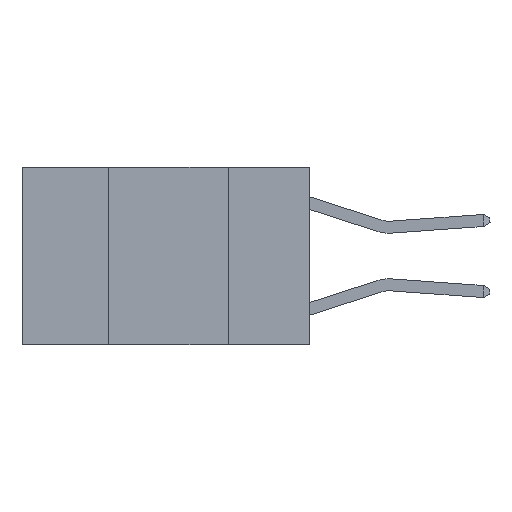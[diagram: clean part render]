
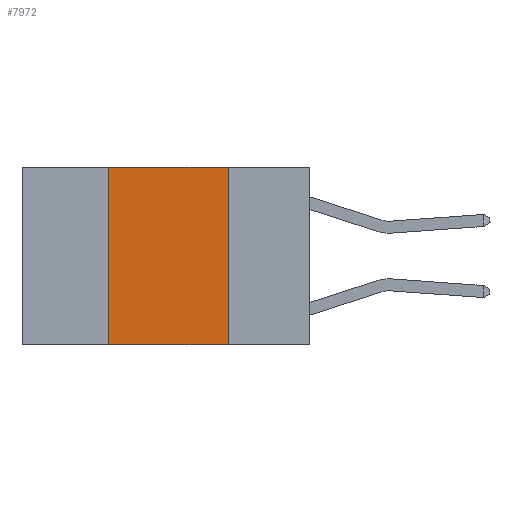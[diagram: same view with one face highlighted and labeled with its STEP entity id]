
A CAD part, left-side view. The second image highlights one B-rep face of the part: STEP entity #7972.
In plain terms, the highlighted planar face has unit normal (-1, 0, 0).
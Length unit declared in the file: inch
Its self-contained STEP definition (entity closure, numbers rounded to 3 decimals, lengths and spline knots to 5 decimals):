
#129 = DIRECTION ( 'NONE',  ( 0., -1., 0. ) ) ;
#263 = CARTESIAN_POINT ( 'NONE',  ( 0., 0.42, 0. ) ) ;
#1276 = VERTEX_POINT ( 'NONE', #3609 ) ;
#1628 = DIRECTION ( 'NONE',  ( 0., 0., -1. ) ) ;
#1835 = LINE ( 'NONE', #263, #6641 ) ;
#2330 = LINE ( 'NONE', #5714, #4734 ) ;
#2497 = AXIS2_PLACEMENT_3D ( 'NONE', #11350, #12351, #6317 ) ;
#3365 = EDGE_CURVE ( 'NONE', #4051, #1276, #8984, .T. ) ;
#3609 = CARTESIAN_POINT ( 'NONE',  ( 0., 0.17, 0. ) ) ;
#3941 = ORIENTED_EDGE ( 'NONE', *, *, #6022, .F. ) ;
#4051 = VERTEX_POINT ( 'NONE', #10719 ) ;
#4151 = VECTOR ( 'NONE', #9758, 39.37008 ) ;
#4244 = PLANE ( 'NONE',  #2497 ) ;
#4476 = EDGE_CURVE ( 'NONE', #4610, #5116, #7010, .T. ) ;
#4610 = VERTEX_POINT ( 'NONE', #5513 ) ;
#4734 = VECTOR ( 'NONE', #1628, 39.37008 ) ;
#5116 = VERTEX_POINT ( 'NONE', #9313 ) ;
#5513 = CARTESIAN_POINT ( 'NONE',  ( 0., 0.42, -0.37 ) ) ;
#5714 = CARTESIAN_POINT ( 'NONE',  ( 0., 0.17, 0. ) ) ;
#6022 = EDGE_CURVE ( 'NONE', #1276, #5116, #2330, .T. ) ;
#6282 = ORIENTED_EDGE ( 'NONE', *, *, #4476, .T. ) ;
#6317 = DIRECTION ( 'NONE',  ( 0., 0., -1. ) ) ;
#6641 = VECTOR ( 'NONE', #7443, 39.37008 ) ;
#6689 = VECTOR ( 'NONE', #129, 39.37008 ) ;
#7010 = LINE ( 'NONE', #9363, #6689 ) ;
#7443 = DIRECTION ( 'NONE',  ( 0., 0., 1. ) ) ;
#7972 = ADVANCED_FACE ( 'NONE', ( #8951 ), #4244, .F. ) ;
#8773 = EDGE_CURVE ( 'NONE', #4610, #4051, #1835, .T. ) ;
#8842 = ORIENTED_EDGE ( 'NONE', *, *, #8773, .F. ) ;
#8951 = FACE_OUTER_BOUND ( 'NONE', #12488, .T. ) ;
#8984 = LINE ( 'NONE', #9839, #4151 ) ;
#9313 = CARTESIAN_POINT ( 'NONE',  ( 0., 0.17, -0.37 ) ) ;
#9363 = CARTESIAN_POINT ( 'NONE',  ( 0., 0.6, -0.37 ) ) ;
#9758 = DIRECTION ( 'NONE',  ( 0., -1., 0. ) ) ;
#9839 = CARTESIAN_POINT ( 'NONE',  ( 0., 0.6, 0. ) ) ;
#10578 = ORIENTED_EDGE ( 'NONE', *, *, #3365, .F. ) ;
#10719 = CARTESIAN_POINT ( 'NONE',  ( 0., 0.42, 0. ) ) ;
#11350 = CARTESIAN_POINT ( 'NONE',  ( 0., 0.6, 0. ) ) ;
#12351 = DIRECTION ( 'NONE',  ( 1., 0., 0. ) ) ;
#12488 = EDGE_LOOP ( 'NONE', ( #3941, #10578, #8842, #6282 ) ) ;
